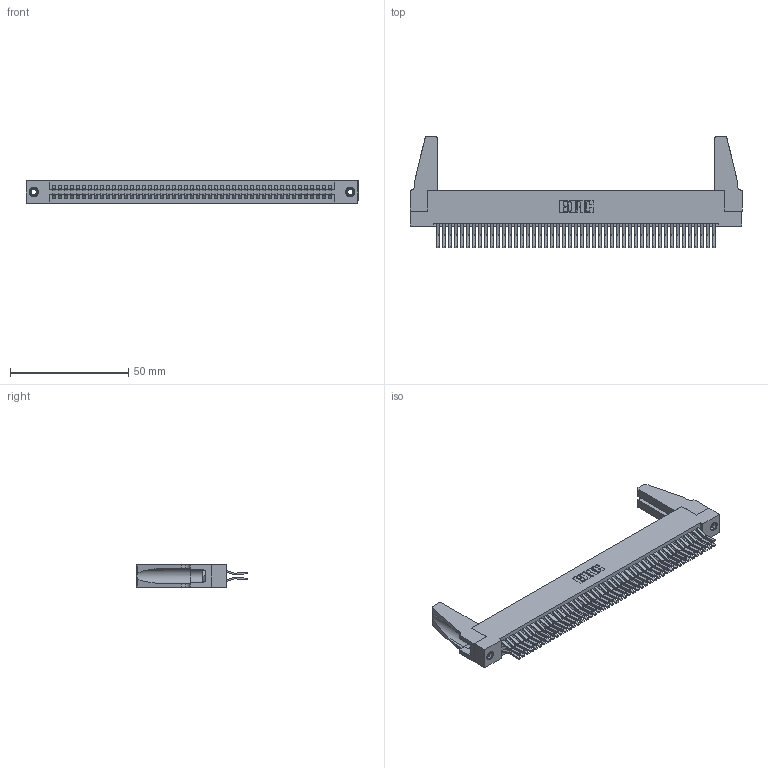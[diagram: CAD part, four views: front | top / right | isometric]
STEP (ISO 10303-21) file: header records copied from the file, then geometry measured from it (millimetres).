
FILE_DESCRIPTION (( 'STEP AP203' ), '1' );
FILE_NAME ('345-094-560-288.STEP', '2019-11-02T06:17:34', ( '' ), ( '' ), 'SwSTEP 2.0', 'SolidWorks 2016', '' );
FILE_SCHEMA (( 'CONFIG_CONTROL_DESIGN' ));
Length unit declared in the file: inch
Products named in the file (5): 345 Part_Flush Mounting Lugs - 0.156 Dia-TH; 345-220-078_345-220-088; 345-094-560-288; 345-250-001_345-250-001-102; 345-292-001_560 Tail
Assembly tree (99 placements, depth 2):
  345-094-560-288
    345 Part_Flush Mounting Lugs - 0.156 Dia-TH
    345-292-001_560 Tail  x94
    345-250-001_345-250-001-102  x2
    345-220-078_345-220-088  x2
Bounding box: 140.61 x 47.31 x 9.4 mm (x, y, z)
Volume: 17574.4 mm3; surface area: 25973.9 mm2
Topology: 99 solids, 99 shells, 5138 faces, 15225 edges, 10014 vertices
Faces by surface type: plane 3254, cylinder 1868, cone 12, torus 4
Entity records: 38440 total; most frequent: CARTESIAN_POINT 6434, ORIENTED_EDGE 6328, DIRECTION 5676, EDGE_CURVE 3164, LINE 2798, VECTOR 2798, VERTEX_POINT 2102, AXIS2_PLACEMENT_3D 1439
